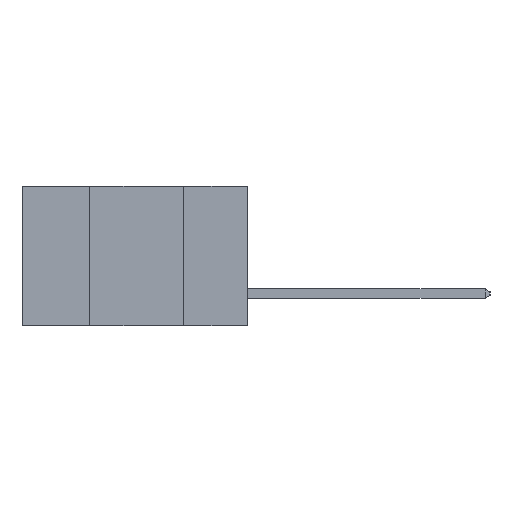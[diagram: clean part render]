
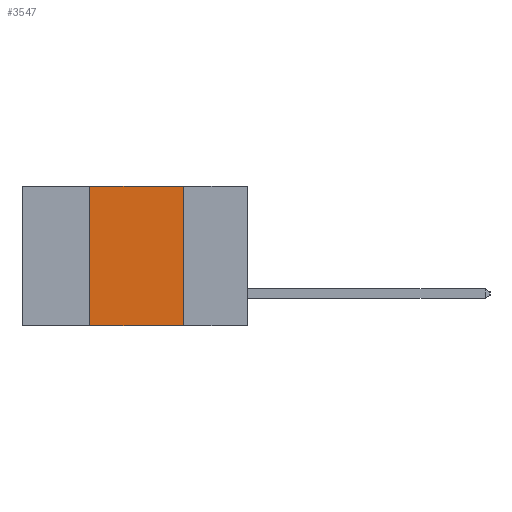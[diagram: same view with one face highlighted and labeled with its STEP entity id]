
A CAD part, left-side view. The second image highlights one B-rep face of the part: STEP entity #3547.
In plain terms, the highlighted planar face has unit normal (-1, 0, 0).
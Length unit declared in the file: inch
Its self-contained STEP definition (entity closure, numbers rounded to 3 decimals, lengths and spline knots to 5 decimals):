
#25 = VERTEX_POINT ( 'NONE', #14996 ) ;
#267 = CARTESIAN_POINT ( 'NONE',  ( 0., 0.6, 0. ) ) ;
#543 = CARTESIAN_POINT ( 'NONE',  ( 0., 0.17, 0. ) ) ;
#1146 = ORIENTED_EDGE ( 'NONE', *, *, #5309, .F. ) ;
#1831 = VECTOR ( 'NONE', #14631, 39.37008 ) ;
#1967 = CARTESIAN_POINT ( 'NONE',  ( 0., 0.42, 0. ) ) ;
#2029 = DIRECTION ( 'NONE',  ( 0., -1., 0. ) ) ;
#2975 = EDGE_CURVE ( 'NONE', #21010, #25, #19821, .T. ) ;
#3547 = ADVANCED_FACE ( 'NONE', ( #11874 ), #13672, .F. ) ;
#3740 = DIRECTION ( 'NONE',  ( 0., 0., 1. ) ) ;
#3826 = CARTESIAN_POINT ( 'NONE',  ( 0., 0.6, -0.37 ) ) ;
#4967 = ORIENTED_EDGE ( 'NONE', *, *, #18437, .F. ) ;
#5309 = EDGE_CURVE ( 'NONE', #21010, #7994, #6287, .T. ) ;
#5722 = VECTOR ( 'NONE', #3740, 39.37008 ) ;
#6287 = LINE ( 'NONE', #1967, #5722 ) ;
#7048 = CARTESIAN_POINT ( 'NONE',  ( 0., 0.42, -0.37 ) ) ;
#7321 = VERTEX_POINT ( 'NONE', #13945 ) ;
#7994 = VERTEX_POINT ( 'NONE', #17359 ) ;
#9495 = DIRECTION ( 'NONE',  ( 1., 0., 0. ) ) ;
#9806 = DIRECTION ( 'NONE',  ( 0., -1., 0. ) ) ;
#10056 = AXIS2_PLACEMENT_3D ( 'NONE', #13332, #9495, #10550 ) ;
#10535 = VECTOR ( 'NONE', #9806, 39.37008 ) ;
#10550 = DIRECTION ( 'NONE',  ( 0., 0., -1. ) ) ;
#10974 = VECTOR ( 'NONE', #2029, 39.37008 ) ;
#11229 = LINE ( 'NONE', #543, #1831 ) ;
#11874 = FACE_OUTER_BOUND ( 'NONE', #21889, .T. ) ;
#13332 = CARTESIAN_POINT ( 'NONE',  ( 0., 0.6, 0. ) ) ;
#13539 = ORIENTED_EDGE ( 'NONE', *, *, #13827, .F. ) ;
#13672 = PLANE ( 'NONE',  #10056 ) ;
#13827 = EDGE_CURVE ( 'NONE', #7994, #7321, #14522, .T. ) ;
#13945 = CARTESIAN_POINT ( 'NONE',  ( 0., 0.17, 0. ) ) ;
#14522 = LINE ( 'NONE', #267, #10974 ) ;
#14631 = DIRECTION ( 'NONE',  ( 0., 0., -1. ) ) ;
#14996 = CARTESIAN_POINT ( 'NONE',  ( 0., 0.17, -0.37 ) ) ;
#17359 = CARTESIAN_POINT ( 'NONE',  ( 0., 0.42, 0. ) ) ;
#18437 = EDGE_CURVE ( 'NONE', #7321, #25, #11229, .T. ) ;
#19821 = LINE ( 'NONE', #3826, #10535 ) ;
#20370 = ORIENTED_EDGE ( 'NONE', *, *, #2975, .T. ) ;
#21010 = VERTEX_POINT ( 'NONE', #7048 ) ;
#21889 = EDGE_LOOP ( 'NONE', ( #4967, #13539, #1146, #20370 ) ) ;
